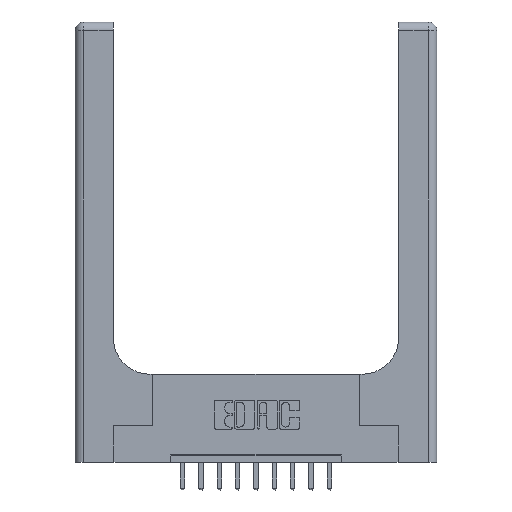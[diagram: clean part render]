
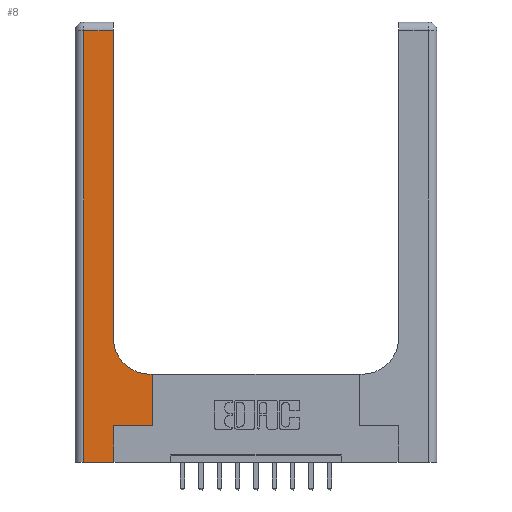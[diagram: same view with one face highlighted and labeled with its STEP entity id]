
A CAD part, top view. The second image highlights one B-rep face of the part: STEP entity #8.
In plain terms, the highlighted planar face has unit normal (0, 0, 1).
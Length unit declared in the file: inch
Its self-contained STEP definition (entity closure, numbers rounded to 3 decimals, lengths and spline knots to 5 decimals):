
#8 = ADVANCED_FACE ( 'NONE', ( #6756 ), #7880, .F. ) ;
#975 = ORIENTED_EDGE ( 'NONE', *, *, #11479, .T. ) ;
#1081 = ORIENTED_EDGE ( 'NONE', *, *, #11275, .T. ) ;
#1158 = VERTEX_POINT ( 'NONE', #6931 ) ;
#1267 = CARTESIAN_POINT ( 'NONE',  ( 0.265, 0., 0.37 ) ) ;
#1354 = VECTOR ( 'NONE', #5765, 39.37008 ) ;
#1465 = EDGE_CURVE ( 'NONE', #14117, #3991, #9926, .T. ) ;
#1582 = EDGE_LOOP ( 'NONE', ( #5247, #8464, #1081, #11883, #4935, #975, #7745, #12978, #15128 ) ) ;
#2013 = EDGE_CURVE ( 'NONE', #5553, #4348, #12246, .T. ) ;
#2055 = CARTESIAN_POINT ( 'NONE',  ( 0.26, 0.85, 0.37 ) ) ;
#2195 = VECTOR ( 'NONE', #10966, 39.37008 ) ;
#2483 = CARTESIAN_POINT ( 'NONE',  ( 0.26, 3., 0.37 ) ) ;
#2487 = CARTESIAN_POINT ( 'NONE',  ( 0.528, 0.25, 0.37 ) ) ;
#3260 = LINE ( 'NONE', #6807, #1354 ) ;
#3376 = CARTESIAN_POINT ( 'NONE',  ( 0.26, 0.6, 0.37 ) ) ;
#3411 = DIRECTION ( 'NONE',  ( 1., 0., 0. ) ) ;
#3490 = CARTESIAN_POINT ( 'NONE',  ( 0.26, 2.94, 0.37 ) ) ;
#3562 = DIRECTION ( 'NONE',  ( 0., 0., -1. ) ) ;
#3991 = VERTEX_POINT ( 'NONE', #13195 ) ;
#4240 = VERTEX_POINT ( 'NONE', #6362 ) ;
#4348 = VERTEX_POINT ( 'NONE', #14431 ) ;
#4843 = EDGE_CURVE ( 'NONE', #10298, #5553, #7371, .T. ) ;
#4875 = DIRECTION ( 'NONE',  ( 0., 1., 0. ) ) ;
#4935 = ORIENTED_EDGE ( 'NONE', *, *, #12382, .T. ) ;
#5247 = ORIENTED_EDGE ( 'NONE', *, *, #4843, .T. ) ;
#5553 = VERTEX_POINT ( 'NONE', #3490 ) ;
#5630 = DIRECTION ( 'NONE',  ( 1., 0., 0. ) ) ;
#5765 = DIRECTION ( 'NONE',  ( 1., 0., 0. ) ) ;
#6362 = CARTESIAN_POINT ( 'NONE',  ( 0.265, 0.25, 0.37 ) ) ;
#6756 = FACE_OUTER_BOUND ( 'NONE', #1582, .T. ) ;
#6807 = CARTESIAN_POINT ( 'NONE',  ( 0.265, 0.25, 0.37 ) ) ;
#6931 = CARTESIAN_POINT ( 'NONE',  ( 0.06, 0., 0.37 ) ) ;
#6956 = VECTOR ( 'NONE', #14715, 39.37008 ) ;
#6993 = VECTOR ( 'NONE', #9377, 39.37008 ) ;
#7371 = LINE ( 'NONE', #2483, #15189 ) ;
#7745 = ORIENTED_EDGE ( 'NONE', *, *, #1465, .T. ) ;
#7880 = PLANE ( 'NONE',  #12904 ) ;
#8050 = DIRECTION ( 'NONE',  ( 0., 0., -1. ) ) ;
#8464 = ORIENTED_EDGE ( 'NONE', *, *, #2013, .T. ) ;
#8574 = CARTESIAN_POINT ( 'NONE',  ( 0.51, 0.6, 0.37 ) ) ;
#8604 = EDGE_CURVE ( 'NONE', #3991, #15691, #10687, .T. ) ;
#8692 = VECTOR ( 'NONE', #5630, 39.37008 ) ;
#8910 = EDGE_CURVE ( 'NONE', #1158, #10411, #14345, .T. ) ;
#9377 = DIRECTION ( 'NONE',  ( 0., 1., 0. ) ) ;
#9386 = CARTESIAN_POINT ( 'NONE',  ( 0., 3., 0.37 ) ) ;
#9452 = CARTESIAN_POINT ( 'NONE',  ( 0., 0., 0.37 ) ) ;
#9920 = CARTESIAN_POINT ( 'NONE',  ( 0.06, 3., 0.37 ) ) ;
#9926 = LINE ( 'NONE', #2487, #13938 ) ;
#10298 = VERTEX_POINT ( 'NONE', #2055 ) ;
#10411 = VERTEX_POINT ( 'NONE', #1267 ) ;
#10553 = AXIS2_PLACEMENT_3D ( 'NONE', #13289, #3562, #3411 ) ;
#10687 = LINE ( 'NONE', #3376, #14551 ) ;
#10966 = DIRECTION ( 'NONE',  ( -1., 0., 0. ) ) ;
#11046 = CIRCLE ( 'NONE', #10553, 0.25 ) ;
#11275 = EDGE_CURVE ( 'NONE', #4348, #1158, #15763, .T. ) ;
#11479 = EDGE_CURVE ( 'NONE', #4240, #14117, #3260, .T. ) ;
#11673 = EDGE_CURVE ( 'NONE', #15691, #10298, #11046, .T. ) ;
#11813 = DIRECTION ( 'NONE',  ( -1., 0., 0. ) ) ;
#11883 = ORIENTED_EDGE ( 'NONE', *, *, #8910, .T. ) ;
#12246 = LINE ( 'NONE', #14856, #2195 ) ;
#12251 = DIRECTION ( 'NONE',  ( 0., 1., 0. ) ) ;
#12382 = EDGE_CURVE ( 'NONE', #10411, #4240, #13158, .T. ) ;
#12904 = AXIS2_PLACEMENT_3D ( 'NONE', #9386, #8050, #15449 ) ;
#12978 = ORIENTED_EDGE ( 'NONE', *, *, #8604, .T. ) ;
#13158 = LINE ( 'NONE', #14417, #6993 ) ;
#13195 = CARTESIAN_POINT ( 'NONE',  ( 0.528, 0.6, 0.37 ) ) ;
#13289 = CARTESIAN_POINT ( 'NONE',  ( 0.51, 0.85, 0.37 ) ) ;
#13938 = VECTOR ( 'NONE', #4875, 39.37008 ) ;
#13943 = CARTESIAN_POINT ( 'NONE',  ( 0.528, 0.25, 0.37 ) ) ;
#14117 = VERTEX_POINT ( 'NONE', #13943 ) ;
#14345 = LINE ( 'NONE', #9452, #8692 ) ;
#14417 = CARTESIAN_POINT ( 'NONE',  ( 0.265, 0., 0.37 ) ) ;
#14431 = CARTESIAN_POINT ( 'NONE',  ( 0.06, 2.94, 0.37 ) ) ;
#14551 = VECTOR ( 'NONE', #11813, 39.37008 ) ;
#14715 = DIRECTION ( 'NONE',  ( 0., -1., 0. ) ) ;
#14856 = CARTESIAN_POINT ( 'NONE',  ( 0., 2.94, 0.37 ) ) ;
#15128 = ORIENTED_EDGE ( 'NONE', *, *, #11673, .T. ) ;
#15189 = VECTOR ( 'NONE', #12251, 39.37008 ) ;
#15449 = DIRECTION ( 'NONE',  ( -1., 0., 0. ) ) ;
#15691 = VERTEX_POINT ( 'NONE', #8574 ) ;
#15763 = LINE ( 'NONE', #9920, #6956 ) ;
